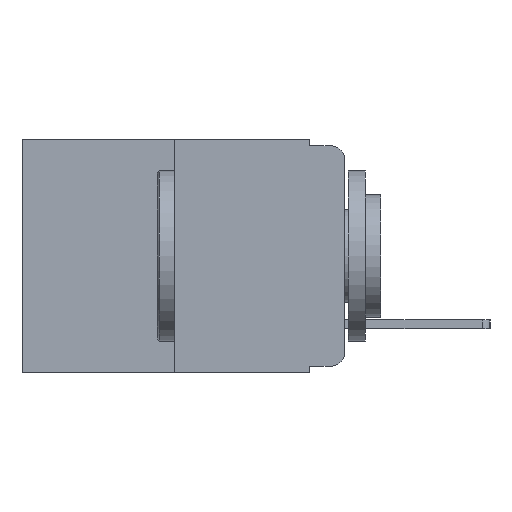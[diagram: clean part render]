
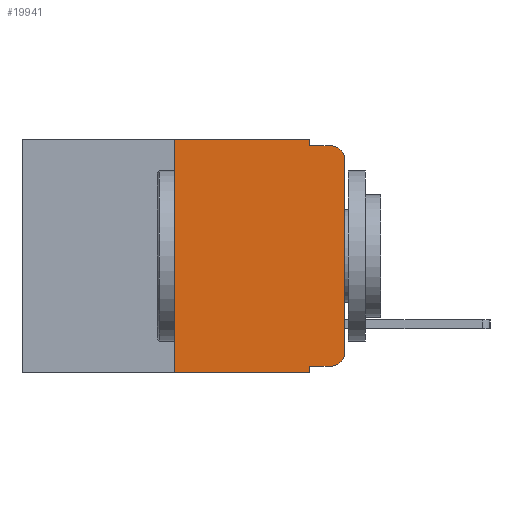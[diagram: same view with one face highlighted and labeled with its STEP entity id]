
A CAD part, left-side view. The second image highlights one B-rep face of the part: STEP entity #19941.
In plain terms, the highlighted planar face has unit normal (-1, 0, 0).
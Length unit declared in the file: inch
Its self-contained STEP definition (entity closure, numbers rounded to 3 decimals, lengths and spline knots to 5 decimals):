
#41 = CARTESIAN_POINT ( 'NONE',  ( 0., 0., -0.313 ) ) ;
#397 = EDGE_CURVE ( 'NONE', #6630, #8199, #18759, .T. ) ;
#1025 = LINE ( 'NONE', #18422, #18087 ) ;
#1051 = VERTEX_POINT ( 'NONE', #20317 ) ;
#1218 = LINE ( 'NONE', #11913, #9488 ) ;
#1335 = DIRECTION ( 'NONE',  ( 0., 0., 1. ) ) ;
#1438 = ORIENTED_EDGE ( 'NONE', *, *, #17500, .F. ) ;
#1461 = EDGE_CURVE ( 'NONE', #16620, #9382, #20031, .T. ) ;
#2540 = VECTOR ( 'NONE', #1335, 39.37008 ) ;
#2606 = CARTESIAN_POINT ( 'NONE',  ( 0., 0.051, 0. ) ) ;
#2692 = CARTESIAN_POINT ( 'NONE',  ( 0., 0.051, 0. ) ) ;
#2772 = ORIENTED_EDGE ( 'NONE', *, *, #13587, .F. ) ;
#2865 = DIRECTION ( 'NONE',  ( -1., 0., 0. ) ) ;
#3016 = DIRECTION ( 'NONE',  ( 0., -1., 0. ) ) ;
#3522 = VECTOR ( 'NONE', #3016, 39.37008 ) ;
#4211 = LINE ( 'NONE', #2692, #12398 ) ;
#4471 = LINE ( 'NONE', #11125, #20946 ) ;
#4729 = CARTESIAN_POINT ( 'NONE',  ( 0., 0.473, 0. ) ) ;
#4950 = DIRECTION ( 'NONE',  ( 0., 0., -1. ) ) ;
#5175 = VERTEX_POINT ( 'NONE', #15566 ) ;
#5188 = ORIENTED_EDGE ( 'NONE', *, *, #7688, .F. ) ;
#5347 = DIRECTION ( 'NONE',  ( -1., 0., 0. ) ) ;
#6245 = CARTESIAN_POINT ( 'NONE',  ( 0., 0.051, -0.01 ) ) ;
#6425 = CIRCLE ( 'NONE', #16280, 0.02 ) ;
#6459 = EDGE_CURVE ( 'NONE', #19553, #11840, #6425, .T. ) ;
#6584 = CARTESIAN_POINT ( 'NONE',  ( 0., 0.473, -0.343 ) ) ;
#6594 = EDGE_LOOP ( 'NONE', ( #20991, #18237, #18868, #1438, #5188, #2772, #9047, #16807, #16403, #15812 ) ) ;
#6630 = VERTEX_POINT ( 'NONE', #14797 ) ;
#6959 = LINE ( 'NONE', #12868, #2540 ) ;
#7331 = FACE_OUTER_BOUND ( 'NONE', #6594, .T. ) ;
#7688 = EDGE_CURVE ( 'NONE', #8606, #12506, #8924, .T. ) ;
#8199 = VERTEX_POINT ( 'NONE', #14268 ) ;
#8232 = DIRECTION ( 'NONE',  ( 0., -1., 0. ) ) ;
#8606 = VERTEX_POINT ( 'NONE', #8829 ) ;
#8775 = AXIS2_PLACEMENT_3D ( 'NONE', #15163, #5347, #16814 ) ;
#8829 = CARTESIAN_POINT ( 'NONE',  ( 0., 0.25, 0. ) ) ;
#8924 = LINE ( 'NONE', #4729, #3522 ) ;
#9047 = ORIENTED_EDGE ( 'NONE', *, *, #397, .T. ) ;
#9050 = CIRCLE ( 'NONE', #8775, 0.02 ) ;
#9382 = VERTEX_POINT ( 'NONE', #14088 ) ;
#9488 = VECTOR ( 'NONE', #13579, 39.37008 ) ;
#9494 = EDGE_CURVE ( 'NONE', #1051, #19553, #4471, .T. ) ;
#10013 = VECTOR ( 'NONE', #8232, 39.37008 ) ;
#10155 = EDGE_CURVE ( 'NONE', #5175, #9382, #9050, .T. ) ;
#10425 = EDGE_CURVE ( 'NONE', #1051, #8199, #4211, .T. ) ;
#10699 = VECTOR ( 'NONE', #18896, 39.37008 ) ;
#11125 = CARTESIAN_POINT ( 'NONE',  ( 0., 0.051, -0.333 ) ) ;
#11438 = CARTESIAN_POINT ( 'NONE',  ( 0., 0.473, 0. ) ) ;
#11840 = VERTEX_POINT ( 'NONE', #41 ) ;
#11913 = CARTESIAN_POINT ( 'NONE',  ( 0., 0.25, 0. ) ) ;
#12398 = VECTOR ( 'NONE', #17537, 39.37008 ) ;
#12506 = VERTEX_POINT ( 'NONE', #2606 ) ;
#12573 = AXIS2_PLACEMENT_3D ( 'NONE', #11438, #14758, #4950 ) ;
#12715 = CARTESIAN_POINT ( 'NONE',  ( 0., 0.02, -0.313 ) ) ;
#12791 = DIRECTION ( 'NONE',  ( 0., -1., 0. ) ) ;
#12868 = CARTESIAN_POINT ( 'NONE',  ( 0., 0., 0. ) ) ;
#13107 = PLANE ( 'NONE',  #12573 ) ;
#13296 = EDGE_CURVE ( 'NONE', #11840, #5175, #6959, .T. ) ;
#13579 = DIRECTION ( 'NONE',  ( 0., 0., 1. ) ) ;
#13587 = EDGE_CURVE ( 'NONE', #6630, #8606, #1218, .T. ) ;
#14088 = CARTESIAN_POINT ( 'NONE',  ( 0., 0.02, -0.01 ) ) ;
#14268 = CARTESIAN_POINT ( 'NONE',  ( 0., 0.051, -0.343 ) ) ;
#14363 = DIRECTION ( 'NONE',  ( 0., 0., -1. ) ) ;
#14758 = DIRECTION ( 'NONE',  ( 1., 0., 0. ) ) ;
#14797 = CARTESIAN_POINT ( 'NONE',  ( 0., 0.25, -0.343 ) ) ;
#15163 = CARTESIAN_POINT ( 'NONE',  ( 0., 0.02, -0.03 ) ) ;
#15566 = CARTESIAN_POINT ( 'NONE',  ( 0., 0., -0.03 ) ) ;
#15812 = ORIENTED_EDGE ( 'NONE', *, *, #6459, .T. ) ;
#16280 = AXIS2_PLACEMENT_3D ( 'NONE', #12715, #2865, #14363 ) ;
#16403 = ORIENTED_EDGE ( 'NONE', *, *, #9494, .T. ) ;
#16620 = VERTEX_POINT ( 'NONE', #6245 ) ;
#16749 = DIRECTION ( 'NONE',  ( 0., 0., -1. ) ) ;
#16807 = ORIENTED_EDGE ( 'NONE', *, *, #10425, .F. ) ;
#16814 = DIRECTION ( 'NONE',  ( 0., 0., -1. ) ) ;
#17221 = CARTESIAN_POINT ( 'NONE',  ( 0., 0.051, -0.01 ) ) ;
#17500 = EDGE_CURVE ( 'NONE', #12506, #16620, #1025, .T. ) ;
#17537 = DIRECTION ( 'NONE',  ( 0., 0., -1. ) ) ;
#18087 = VECTOR ( 'NONE', #16749, 39.37008 ) ;
#18237 = ORIENTED_EDGE ( 'NONE', *, *, #10155, .T. ) ;
#18422 = CARTESIAN_POINT ( 'NONE',  ( 0., 0.051, 0. ) ) ;
#18759 = LINE ( 'NONE', #6584, #10013 ) ;
#18810 = CARTESIAN_POINT ( 'NONE',  ( 0., 0.02, -0.333 ) ) ;
#18868 = ORIENTED_EDGE ( 'NONE', *, *, #1461, .F. ) ;
#18896 = DIRECTION ( 'NONE',  ( 0., -1., 0. ) ) ;
#19553 = VERTEX_POINT ( 'NONE', #18810 ) ;
#19941 = ADVANCED_FACE ( 'NONE', ( #7331 ), #13107, .F. ) ;
#20031 = LINE ( 'NONE', #17221, #10699 ) ;
#20317 = CARTESIAN_POINT ( 'NONE',  ( 0., 0.051, -0.333 ) ) ;
#20946 = VECTOR ( 'NONE', #12791, 39.37008 ) ;
#20991 = ORIENTED_EDGE ( 'NONE', *, *, #13296, .T. ) ;
